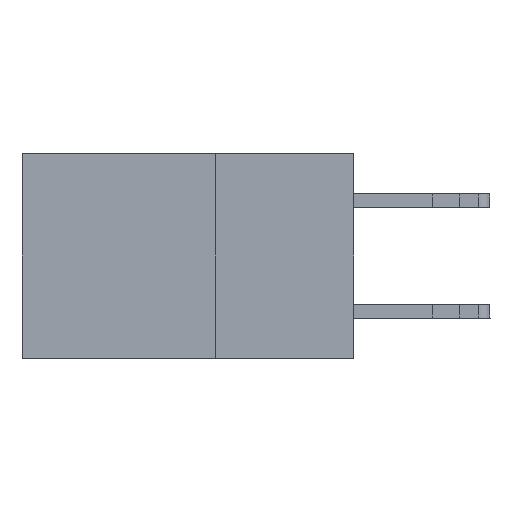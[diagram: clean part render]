
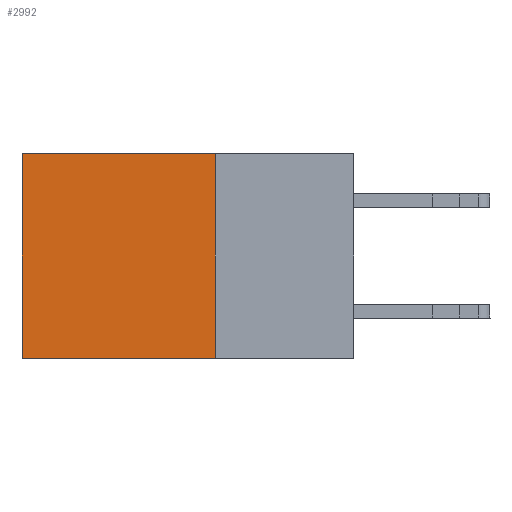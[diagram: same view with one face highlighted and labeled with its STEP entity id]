
A CAD part, left-side view. The second image highlights one B-rep face of the part: STEP entity #2992.
In plain terms, the highlighted planar face has unit normal (-1, 0, 0).
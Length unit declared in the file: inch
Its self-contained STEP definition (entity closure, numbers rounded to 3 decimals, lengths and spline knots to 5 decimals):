
#675 = ORIENTED_EDGE ( 'NONE', *, *, #20766, .T. ) ;
#815 = VERTEX_POINT ( 'NONE', #14900 ) ;
#1228 = VERTEX_POINT ( 'NONE', #4094 ) ;
#1409 = PLANE ( 'NONE',  #21042 ) ;
#1753 = CARTESIAN_POINT ( 'NONE',  ( 0.2875, 0.25, 0. ) ) ;
#2100 = ORIENTED_EDGE ( 'NONE', *, *, #18699, .F. ) ;
#2992 = ADVANCED_FACE ( 'NONE', ( #20984 ), #1409, .F. ) ;
#3752 = LINE ( 'NONE', #1753, #7600 ) ;
#4094 = CARTESIAN_POINT ( 'NONE',  ( 0.2875, 0.25, 0. ) ) ;
#4328 = CARTESIAN_POINT ( 'NONE',  ( 0.2875, 0.6, 0. ) ) ;
#4598 = CARTESIAN_POINT ( 'NONE',  ( 0.2875, 0.6, 0. ) ) ;
#6764 = DIRECTION ( 'NONE',  ( 0., 0., -1. ) ) ;
#6980 = DIRECTION ( 'NONE',  ( 0., 1., 0. ) ) ;
#7511 = ORIENTED_EDGE ( 'NONE', *, *, #17874, .T. ) ;
#7600 = VECTOR ( 'NONE', #8854, 39.37008 ) ;
#7989 = DIRECTION ( 'NONE',  ( 0., 0., -1. ) ) ;
#8366 = VERTEX_POINT ( 'NONE', #13837 ) ;
#8515 = CARTESIAN_POINT ( 'NONE',  ( 0.2875, 0.25, 0. ) ) ;
#8854 = DIRECTION ( 'NONE',  ( 0., 0., -1. ) ) ;
#9113 = VERTEX_POINT ( 'NONE', #4328 ) ;
#10703 = CARTESIAN_POINT ( 'NONE',  ( 0.2875, 0.25, -0.37 ) ) ;
#11004 = VECTOR ( 'NONE', #6980, 39.37008 ) ;
#11341 = LINE ( 'NONE', #18438, #20388 ) ;
#11996 = EDGE_CURVE ( 'NONE', #1228, #8366, #3752, .T. ) ;
#12570 = VECTOR ( 'NONE', #7989, 39.37008 ) ;
#13837 = CARTESIAN_POINT ( 'NONE',  ( 0.2875, 0.25, -0.37 ) ) ;
#14900 = CARTESIAN_POINT ( 'NONE',  ( 0.2875, 0.6, -0.37 ) ) ;
#15685 = DIRECTION ( 'NONE',  ( 1., 0., 0. ) ) ;
#17159 = ORIENTED_EDGE ( 'NONE', *, *, #11996, .F. ) ;
#17874 = EDGE_CURVE ( 'NONE', #1228, #9113, #11341, .T. ) ;
#18438 = CARTESIAN_POINT ( 'NONE',  ( 0.2875, 0.25, 0. ) ) ;
#18667 = DIRECTION ( 'NONE',  ( 0., 1., 0. ) ) ;
#18699 = EDGE_CURVE ( 'NONE', #8366, #815, #23065, .T. ) ;
#19597 = EDGE_LOOP ( 'NONE', ( #675, #2100, #17159, #7511 ) ) ;
#20388 = VECTOR ( 'NONE', #18667, 39.37008 ) ;
#20766 = EDGE_CURVE ( 'NONE', #9113, #815, #22335, .T. ) ;
#20984 = FACE_OUTER_BOUND ( 'NONE', #19597, .T. ) ;
#21042 = AXIS2_PLACEMENT_3D ( 'NONE', #8515, #15685, #6764 ) ;
#22335 = LINE ( 'NONE', #4598, #12570 ) ;
#23065 = LINE ( 'NONE', #10703, #11004 ) ;
